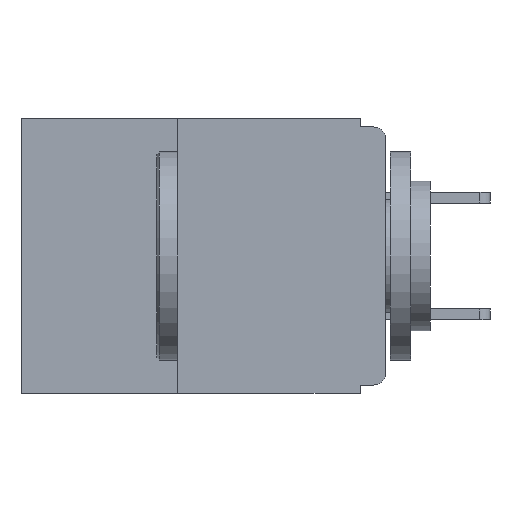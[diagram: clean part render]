
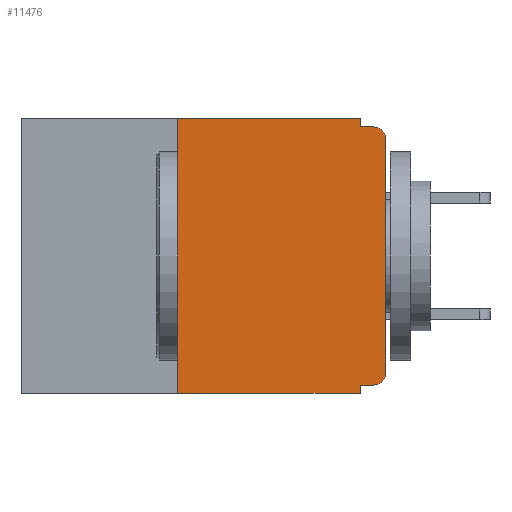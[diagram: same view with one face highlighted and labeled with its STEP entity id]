
A CAD part, left-side view. The second image highlights one B-rep face of the part: STEP entity #11476.
In plain terms, the highlighted planar face has unit normal (-1, 0, 0).
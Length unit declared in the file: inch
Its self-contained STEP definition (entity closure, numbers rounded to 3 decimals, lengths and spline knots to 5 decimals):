
#448 = VERTEX_POINT ( 'NONE', #11935 ) ;
#795 = DIRECTION ( 'NONE',  ( 0., 1., 0. ) ) ;
#817 = DIRECTION ( 'NONE',  ( 0., 0., -1. ) ) ;
#911 = VERTEX_POINT ( 'NONE', #2326 ) ;
#1131 = VERTEX_POINT ( 'NONE', #8031 ) ;
#1148 = VECTOR ( 'NONE', #3949, 39.37008 ) ;
#1150 = VERTEX_POINT ( 'NONE', #9211 ) ;
#1230 = LINE ( 'NONE', #4436, #1148 ) ;
#1254 = CARTESIAN_POINT ( 'NONE',  ( 0., 0., -0.32 ) ) ;
#1277 = VERTEX_POINT ( 'NONE', #7924 ) ;
#1380 = VERTEX_POINT ( 'NONE', #12820 ) ;
#1499 = VERTEX_POINT ( 'NONE', #13074 ) ;
#1868 = CARTESIAN_POINT ( 'NONE',  ( 0., 0.031, -0.33 ) ) ;
#1903 = EDGE_LOOP ( 'NONE', ( #7277, #7624, #7772, #8832, #9143, #10039, #10052, #10453, #10469, #11760 ) ) ;
#2326 = CARTESIAN_POINT ( 'NONE',  ( 0., 0.015, -0.01 ) ) ;
#2401 = VECTOR ( 'NONE', #12038, 39.37008 ) ;
#2427 = LINE ( 'NONE', #12059, #2401 ) ;
#2476 = DIRECTION ( 'NONE',  ( 0., 0., -1. ) ) ;
#2720 = DIRECTION ( 'NONE',  ( -1., 0., 0. ) ) ;
#2783 = CIRCLE ( 'NONE', #12485, 0.015 ) ;
#2870 = CARTESIAN_POINT ( 'NONE',  ( 0., 0.015, -0.025 ) ) ;
#3137 = CARTESIAN_POINT ( 'NONE',  ( 0., 0.25, -0.33 ) ) ;
#3398 = VERTEX_POINT ( 'NONE', #3137 ) ;
#3462 = AXIS2_PLACEMENT_3D ( 'NONE', #2870, #2720, #2476 ) ;
#3919 = VECTOR ( 'NONE', #795, 39.37008 ) ;
#3949 = DIRECTION ( 'NONE',  ( 0., -1., 0. ) ) ;
#4436 = CARTESIAN_POINT ( 'NONE',  ( 0., 0., -0.01 ) ) ;
#4642 = AXIS2_PLACEMENT_3D ( 'NONE', #8054, #7663, #7609 ) ;
#5272 = EDGE_CURVE ( 'NONE', #1380, #1499, #2427, .T. ) ;
#6206 = VECTOR ( 'NONE', #9590, 39.37008 ) ;
#6532 = CARTESIAN_POINT ( 'NONE',  ( 0., 0.031, 0. ) ) ;
#6613 = CARTESIAN_POINT ( 'NONE',  ( 0., 0.437, -0.33 ) ) ;
#6865 = LINE ( 'NONE', #9695, #6206 ) ;
#6991 = DIRECTION ( 'NONE',  ( 0., 0., -1. ) ) ;
#7009 = DIRECTION ( 'NONE',  ( -1., 0., 0. ) ) ;
#7080 = CARTESIAN_POINT ( 'NONE',  ( 0., 0.015, -0.305 ) ) ;
#7102 = VERTEX_POINT ( 'NONE', #12830 ) ;
#7178 = DIRECTION ( 'NONE',  ( 0., 0., -1. ) ) ;
#7277 = ORIENTED_EDGE ( 'NONE', *, *, #5272, .T. ) ;
#7421 = EDGE_CURVE ( 'NONE', #1131, #911, #1230, .T. ) ;
#7609 = DIRECTION ( 'NONE',  ( 0., 0., -1. ) ) ;
#7624 = ORIENTED_EDGE ( 'NONE', *, *, #9220, .T. ) ;
#7663 = DIRECTION ( 'NONE',  ( 1., 0., 0. ) ) ;
#7772 = ORIENTED_EDGE ( 'NONE', *, *, #7421, .F. ) ;
#7796 = VECTOR ( 'NONE', #817, 39.37008 ) ;
#7809 = LINE ( 'NONE', #1868, #7796 ) ;
#7835 = DIRECTION ( 'NONE',  ( 0., -1., 0. ) ) ;
#7924 = CARTESIAN_POINT ( 'NONE',  ( 0., 0.031, -0.32 ) ) ;
#7926 = EDGE_CURVE ( 'NONE', #10441, #7102, #6865, .T. ) ;
#8031 = CARTESIAN_POINT ( 'NONE',  ( 0., 0.031, -0.01 ) ) ;
#8054 = CARTESIAN_POINT ( 'NONE',  ( 0., 0.437, 0. ) ) ;
#8185 = LINE ( 'NONE', #1254, #3919 ) ;
#8349 = EDGE_CURVE ( 'NONE', #1150, #1277, #8185, .T. ) ;
#8631 = PLANE ( 'NONE',  #4642 ) ;
#8832 = ORIENTED_EDGE ( 'NONE', *, *, #11491, .F. ) ;
#9069 = DIRECTION ( 'NONE',  ( 0., 0., 1. ) ) ;
#9143 = ORIENTED_EDGE ( 'NONE', *, *, #7926, .F. ) ;
#9157 = VECTOR ( 'NONE', #7835, 39.37008 ) ;
#9162 = CARTESIAN_POINT ( 'NONE',  ( 0., 0.25, -0.33 ) ) ;
#9191 = LINE ( 'NONE', #6613, #9157 ) ;
#9211 = CARTESIAN_POINT ( 'NONE',  ( 0., 0.015, -0.32 ) ) ;
#9220 = EDGE_CURVE ( 'NONE', #1499, #911, #10270, .T. ) ;
#9590 = DIRECTION ( 'NONE',  ( 0., -1., 0. ) ) ;
#9638 = LINE ( 'NONE', #9162, #9661 ) ;
#9661 = VECTOR ( 'NONE', #9069, 39.37008 ) ;
#9695 = CARTESIAN_POINT ( 'NONE',  ( 0., 0.437, 0. ) ) ;
#10039 = ORIENTED_EDGE ( 'NONE', *, *, #11716, .F. ) ;
#10052 = ORIENTED_EDGE ( 'NONE', *, *, #11888, .T. ) ;
#10249 = EDGE_CURVE ( 'NONE', #1150, #1380, #2783, .T. ) ;
#10270 = CIRCLE ( 'NONE', #3462, 0.015 ) ;
#10441 = VERTEX_POINT ( 'NONE', #11930 ) ;
#10453 = ORIENTED_EDGE ( 'NONE', *, *, #12305, .F. ) ;
#10469 = ORIENTED_EDGE ( 'NONE', *, *, #8349, .F. ) ;
#10619 = VECTOR ( 'NONE', #7178, 39.37008 ) ;
#10680 = LINE ( 'NONE', #6532, #10619 ) ;
#10736 = FACE_OUTER_BOUND ( 'NONE', #1903, .T. ) ;
#11476 = ADVANCED_FACE ( 'NONE', ( #10736 ), #8631, .F. ) ;
#11491 = EDGE_CURVE ( 'NONE', #7102, #1131, #10680, .T. ) ;
#11716 = EDGE_CURVE ( 'NONE', #3398, #10441, #9638, .T. ) ;
#11760 = ORIENTED_EDGE ( 'NONE', *, *, #10249, .T. ) ;
#11888 = EDGE_CURVE ( 'NONE', #3398, #448, #9191, .T. ) ;
#11930 = CARTESIAN_POINT ( 'NONE',  ( 0., 0.25, 0. ) ) ;
#11935 = CARTESIAN_POINT ( 'NONE',  ( 0., 0.031, -0.33 ) ) ;
#12038 = DIRECTION ( 'NONE',  ( 0., 0., 1. ) ) ;
#12059 = CARTESIAN_POINT ( 'NONE',  ( 0., 0., 0. ) ) ;
#12305 = EDGE_CURVE ( 'NONE', #1277, #448, #7809, .T. ) ;
#12485 = AXIS2_PLACEMENT_3D ( 'NONE', #7080, #7009, #6991 ) ;
#12820 = CARTESIAN_POINT ( 'NONE',  ( 0., 0., -0.305 ) ) ;
#12830 = CARTESIAN_POINT ( 'NONE',  ( 0., 0.031, 0. ) ) ;
#13074 = CARTESIAN_POINT ( 'NONE',  ( 0., 0., -0.025 ) ) ;
